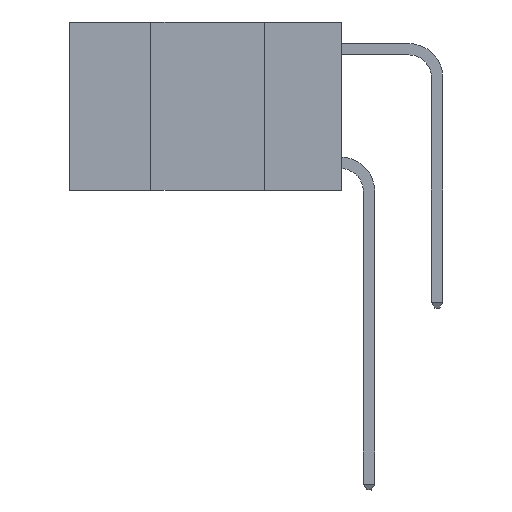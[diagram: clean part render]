
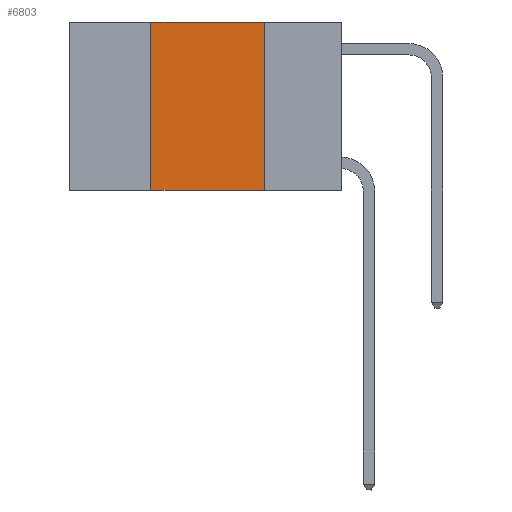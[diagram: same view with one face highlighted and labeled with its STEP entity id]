
A CAD part, left-side view. The second image highlights one B-rep face of the part: STEP entity #6803.
In plain terms, the highlighted planar face has unit normal (-1, 0, 0).
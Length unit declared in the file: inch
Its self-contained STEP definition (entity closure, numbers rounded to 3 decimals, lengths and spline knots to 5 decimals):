
#591 = CARTESIAN_POINT ( 'NONE',  ( 0., 0.42, 0. ) ) ;
#681 = LINE ( 'NONE', #7261, #1997 ) ;
#932 = CARTESIAN_POINT ( 'NONE',  ( 0., 0.42, -0.37 ) ) ;
#1062 = DIRECTION ( 'NONE',  ( 1., 0., 0. ) ) ;
#1619 = DIRECTION ( 'NONE',  ( 0., 0., -1. ) ) ;
#1629 = CARTESIAN_POINT ( 'NONE',  ( 0., 0.6, 0. ) ) ;
#1679 = EDGE_CURVE ( 'NONE', #3699, #4747, #11533, .T. ) ;
#1997 = VECTOR ( 'NONE', #1619, 39.37008 ) ;
#2047 = FACE_OUTER_BOUND ( 'NONE', #4471, .T. ) ;
#2815 = LINE ( 'NONE', #591, #9145 ) ;
#3529 = PLANE ( 'NONE',  #5251 ) ;
#3699 = VERTEX_POINT ( 'NONE', #8231 ) ;
#4471 = EDGE_LOOP ( 'NONE', ( #5055, #9348, #9054, #7814 ) ) ;
#4747 = VERTEX_POINT ( 'NONE', #7071 ) ;
#5055 = ORIENTED_EDGE ( 'NONE', *, *, #10019, .F. ) ;
#5251 = AXIS2_PLACEMENT_3D ( 'NONE', #9427, #1062, #5959 ) ;
#5959 = DIRECTION ( 'NONE',  ( 0., 0., -1. ) ) ;
#6646 = VECTOR ( 'NONE', #7903, 39.37008 ) ;
#6803 = ADVANCED_FACE ( 'NONE', ( #2047 ), #3529, .F. ) ;
#6823 = EDGE_CURVE ( 'NONE', #11106, #3699, #2815, .T. ) ;
#7042 = CARTESIAN_POINT ( 'NONE',  ( 0., 0.6, -0.37 ) ) ;
#7071 = CARTESIAN_POINT ( 'NONE',  ( 0., 0.17, 0. ) ) ;
#7142 = DIRECTION ( 'NONE',  ( 0., -1., 0. ) ) ;
#7255 = VERTEX_POINT ( 'NONE', #9071 ) ;
#7261 = CARTESIAN_POINT ( 'NONE',  ( 0., 0.17, 0. ) ) ;
#7814 = ORIENTED_EDGE ( 'NONE', *, *, #10848, .T. ) ;
#7903 = DIRECTION ( 'NONE',  ( 0., -1., 0. ) ) ;
#8231 = CARTESIAN_POINT ( 'NONE',  ( 0., 0.42, 0. ) ) ;
#8653 = VECTOR ( 'NONE', #7142, 39.37008 ) ;
#9054 = ORIENTED_EDGE ( 'NONE', *, *, #6823, .F. ) ;
#9071 = CARTESIAN_POINT ( 'NONE',  ( 0., 0.17, -0.37 ) ) ;
#9145 = VECTOR ( 'NONE', #9212, 39.37008 ) ;
#9148 = LINE ( 'NONE', #7042, #6646 ) ;
#9212 = DIRECTION ( 'NONE',  ( 0., 0., 1. ) ) ;
#9348 = ORIENTED_EDGE ( 'NONE', *, *, #1679, .F. ) ;
#9427 = CARTESIAN_POINT ( 'NONE',  ( 0., 0.6, 0. ) ) ;
#10019 = EDGE_CURVE ( 'NONE', #4747, #7255, #681, .T. ) ;
#10848 = EDGE_CURVE ( 'NONE', #11106, #7255, #9148, .T. ) ;
#11106 = VERTEX_POINT ( 'NONE', #932 ) ;
#11533 = LINE ( 'NONE', #1629, #8653 ) ;
